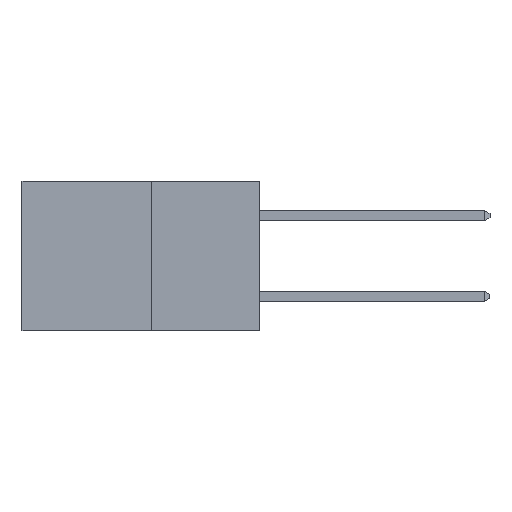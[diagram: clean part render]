
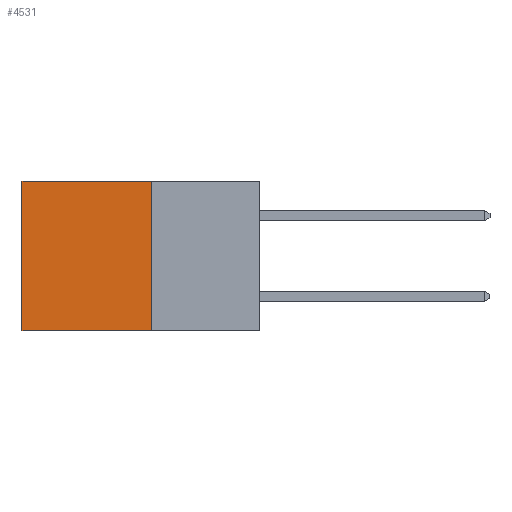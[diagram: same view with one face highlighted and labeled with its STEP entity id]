
A CAD part, left-side view. The second image highlights one B-rep face of the part: STEP entity #4531.
In plain terms, the highlighted planar face has unit normal (-1, 0, 0).
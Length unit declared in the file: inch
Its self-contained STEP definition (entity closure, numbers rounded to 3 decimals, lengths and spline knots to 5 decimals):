
#389 = DIRECTION ( 'NONE',  ( 0., 0., -1. ) ) ;
#643 = AXIS2_PLACEMENT_3D ( 'NONE', #1843, #3754, #7033 ) ;
#699 = CARTESIAN_POINT ( 'NONE',  ( 0.277, 0.27, -0.37 ) ) ;
#1092 = CARTESIAN_POINT ( 'NONE',  ( 0.277, 0.27, -0.37 ) ) ;
#1137 = VECTOR ( 'NONE', #389, 39.37008 ) ;
#1411 = VECTOR ( 'NONE', #6577, 39.37008 ) ;
#1650 = VERTEX_POINT ( 'NONE', #3323 ) ;
#1807 = LINE ( 'NONE', #6557, #1411 ) ;
#1843 = CARTESIAN_POINT ( 'NONE',  ( 0.277, 0.27, -0.37 ) ) ;
#1986 = CARTESIAN_POINT ( 'NONE',  ( 0.277, 0.27, 0. ) ) ;
#2035 = VECTOR ( 'NONE', #5604, 39.37008 ) ;
#2233 = CARTESIAN_POINT ( 'NONE',  ( 0.277, 0.59, 0. ) ) ;
#2808 = FACE_OUTER_BOUND ( 'NONE', #3918, .T. ) ;
#3306 = PLANE ( 'NONE',  #643 ) ;
#3323 = CARTESIAN_POINT ( 'NONE',  ( 0.277, 0.59, -0.37 ) ) ;
#3754 = DIRECTION ( 'NONE',  ( 1., 0., 0. ) ) ;
#3918 = EDGE_LOOP ( 'NONE', ( #5076, #5078, #5318, #5596 ) ) ;
#4266 = VERTEX_POINT ( 'NONE', #1092 ) ;
#4405 = VERTEX_POINT ( 'NONE', #1986 ) ;
#4531 = ADVANCED_FACE ( 'NONE', ( #2808 ), #3306, .F. ) ;
#4649 = EDGE_CURVE ( 'NONE', #4266, #1650, #4929, .T. ) ;
#4929 = LINE ( 'NONE', #5709, #2035 ) ;
#5076 = ORIENTED_EDGE ( 'NONE', *, *, #6477, .T. ) ;
#5078 = ORIENTED_EDGE ( 'NONE', *, *, #4649, .F. ) ;
#5081 = VECTOR ( 'NONE', #6964, 39.37008 ) ;
#5318 = ORIENTED_EDGE ( 'NONE', *, *, #6311, .F. ) ;
#5596 = ORIENTED_EDGE ( 'NONE', *, *, #6418, .T. ) ;
#5604 = DIRECTION ( 'NONE',  ( 0., 1., 0. ) ) ;
#5709 = CARTESIAN_POINT ( 'NONE',  ( 0.277, 0.27, -0.37 ) ) ;
#5813 = VERTEX_POINT ( 'NONE', #2233 ) ;
#6011 = LINE ( 'NONE', #699, #1137 ) ;
#6311 = EDGE_CURVE ( 'NONE', #4405, #4266, #6011, .T. ) ;
#6418 = EDGE_CURVE ( 'NONE', #4405, #5813, #6629, .T. ) ;
#6477 = EDGE_CURVE ( 'NONE', #5813, #1650, #1807, .T. ) ;
#6557 = CARTESIAN_POINT ( 'NONE',  ( 0.277, 0.59, -0.37 ) ) ;
#6577 = DIRECTION ( 'NONE',  ( 0., 0., -1. ) ) ;
#6629 = LINE ( 'NONE', #6993, #5081 ) ;
#6964 = DIRECTION ( 'NONE',  ( 0., 1., 0. ) ) ;
#6993 = CARTESIAN_POINT ( 'NONE',  ( 0.277, 0.27, 0. ) ) ;
#7033 = DIRECTION ( 'NONE',  ( 0., 0., -1. ) ) ;
